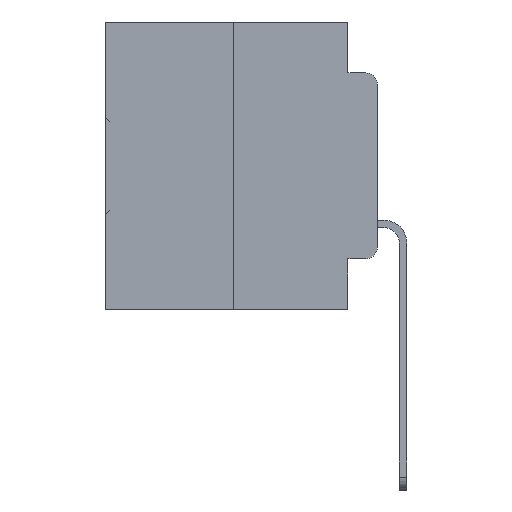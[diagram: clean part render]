
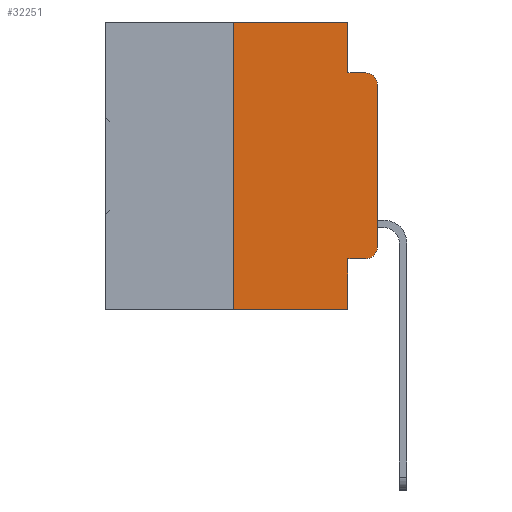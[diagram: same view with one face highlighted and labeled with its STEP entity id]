
A CAD part, left-side view. The second image highlights one B-rep face of the part: STEP entity #32251.
In plain terms, the highlighted planar face has unit normal (-1, 0, 0).
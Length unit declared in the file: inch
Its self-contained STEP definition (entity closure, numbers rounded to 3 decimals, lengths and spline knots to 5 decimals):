
#83 = LINE ( 'NONE', #15399, #19678 ) ;
#830 = ORIENTED_EDGE ( 'NONE', *, *, #25041, .T. ) ;
#836 = CARTESIAN_POINT ( 'NONE',  ( 0., 0.02, -0.3915 ) ) ;
#919 = VERTEX_POINT ( 'NONE', #12145 ) ;
#992 = ORIENTED_EDGE ( 'NONE', *, *, #31967, .T. ) ;
#1198 = VECTOR ( 'NONE', #10958, 39.37008 ) ;
#1769 = EDGE_CURVE ( 'NONE', #11244, #21108, #15442, .T. ) ;
#2056 = DIRECTION ( 'NONE',  ( 0., 0., -1. ) ) ;
#2387 = CARTESIAN_POINT ( 'NONE',  ( 0., 0.051, -0.5 ) ) ;
#3207 = AXIS2_PLACEMENT_3D ( 'NONE', #11219, #29512, #13891 ) ;
#3574 = DIRECTION ( 'NONE',  ( 0., 0., -1. ) ) ;
#4146 = AXIS2_PLACEMENT_3D ( 'NONE', #836, #19469, #3574 ) ;
#4393 = ORIENTED_EDGE ( 'NONE', *, *, #25505, .F. ) ;
#4738 = VECTOR ( 'NONE', #8122, 39.37008 ) ;
#4971 = EDGE_CURVE ( 'NONE', #9365, #25466, #5083, .T. ) ;
#4992 = CARTESIAN_POINT ( 'NONE',  ( 0., 0.051, 0. ) ) ;
#5083 = LINE ( 'NONE', #10403, #18357 ) ;
#5405 = CARTESIAN_POINT ( 'NONE',  ( 0., 0.051, -0.4115 ) ) ;
#8122 = DIRECTION ( 'NONE',  ( 0., -1., 0. ) ) ;
#8273 = CIRCLE ( 'NONE', #4146, 0.02 ) ;
#9365 = VERTEX_POINT ( 'NONE', #17453 ) ;
#10403 = CARTESIAN_POINT ( 'NONE',  ( 0., 0.25, 0. ) ) ;
#10607 = VERTEX_POINT ( 'NONE', #4992 ) ;
#10772 = LINE ( 'NONE', #13073, #17762 ) ;
#10958 = DIRECTION ( 'NONE',  ( 0., 0., 1. ) ) ;
#11066 = EDGE_CURVE ( 'NONE', #9365, #14233, #12855, .T. ) ;
#11219 = CARTESIAN_POINT ( 'NONE',  ( 0., 0.473, 0. ) ) ;
#11244 = VERTEX_POINT ( 'NONE', #16465 ) ;
#11759 = AXIS2_PLACEMENT_3D ( 'NONE', #15131, #33301, #17755 ) ;
#11813 = VECTOR ( 'NONE', #15239, 39.37008 ) ;
#12145 = CARTESIAN_POINT ( 'NONE',  ( 0., 0.02, -0.4115 ) ) ;
#12359 = ORIENTED_EDGE ( 'NONE', *, *, #18378, .F. ) ;
#12530 = CIRCLE ( 'NONE', #11759, 0.02 ) ;
#12855 = LINE ( 'NONE', #20433, #31195 ) ;
#12940 = ORIENTED_EDGE ( 'NONE', *, *, #32003, .F. ) ;
#13073 = CARTESIAN_POINT ( 'NONE',  ( 0., 0.473, 0. ) ) ;
#13258 = EDGE_CURVE ( 'NONE', #10607, #28328, #29925, .T. ) ;
#13891 = DIRECTION ( 'NONE',  ( 0., 0., -1. ) ) ;
#14233 = VERTEX_POINT ( 'NONE', #2387 ) ;
#14582 = ORIENTED_EDGE ( 'NONE', *, *, #1769, .T. ) ;
#15131 = CARTESIAN_POINT ( 'NONE',  ( 0., 0.02, -0.1085 ) ) ;
#15133 = CARTESIAN_POINT ( 'NONE',  ( 0., 0.25, 0. ) ) ;
#15239 = DIRECTION ( 'NONE',  ( 0., -1., 0. ) ) ;
#15251 = VECTOR ( 'NONE', #16353, 39.37008 ) ;
#15399 = CARTESIAN_POINT ( 'NONE',  ( 0., 0.051, 0. ) ) ;
#15442 = LINE ( 'NONE', #21506, #1198 ) ;
#16261 = VERTEX_POINT ( 'NONE', #17396 ) ;
#16353 = DIRECTION ( 'NONE',  ( 0., 0., -1. ) ) ;
#16465 = CARTESIAN_POINT ( 'NONE',  ( 0., 0., -0.3915 ) ) ;
#17396 = CARTESIAN_POINT ( 'NONE',  ( 0., 0.051, -0.4115 ) ) ;
#17453 = CARTESIAN_POINT ( 'NONE',  ( 0., 0.25, -0.5 ) ) ;
#17499 = ORIENTED_EDGE ( 'NONE', *, *, #11066, .T. ) ;
#17755 = DIRECTION ( 'NONE',  ( 0., 0., -1. ) ) ;
#17762 = VECTOR ( 'NONE', #28704, 39.37008 ) ;
#18357 = VECTOR ( 'NONE', #20834, 39.37008 ) ;
#18378 = EDGE_CURVE ( 'NONE', #25466, #10607, #10772, .T. ) ;
#18434 = FACE_OUTER_BOUND ( 'NONE', #30913, .T. ) ;
#19469 = DIRECTION ( 'NONE',  ( -1., 0., 0. ) ) ;
#19678 = VECTOR ( 'NONE', #2056, 39.37008 ) ;
#20121 = ORIENTED_EDGE ( 'NONE', *, *, #4971, .F. ) ;
#20433 = CARTESIAN_POINT ( 'NONE',  ( 0., 0.473, -0.5 ) ) ;
#20779 = ORIENTED_EDGE ( 'NONE', *, *, #23313, .T. ) ;
#20834 = DIRECTION ( 'NONE',  ( 0., 0., 1. ) ) ;
#21108 = VERTEX_POINT ( 'NONE', #25754 ) ;
#21506 = CARTESIAN_POINT ( 'NONE',  ( 0., 0., 0. ) ) ;
#21663 = PLANE ( 'NONE',  #3207 ) ;
#22356 = ORIENTED_EDGE ( 'NONE', *, *, #13258, .F. ) ;
#22930 = DIRECTION ( 'NONE',  ( 0., -1., 0. ) ) ;
#23313 = EDGE_CURVE ( 'NONE', #919, #11244, #8273, .T. ) ;
#24182 = CARTESIAN_POINT ( 'NONE',  ( 0., 0.02, -0.0885 ) ) ;
#25041 = EDGE_CURVE ( 'NONE', #16261, #919, #32653, .T. ) ;
#25466 = VERTEX_POINT ( 'NONE', #15133 ) ;
#25505 = EDGE_CURVE ( 'NONE', #28328, #30477, #31829, .T. ) ;
#25754 = CARTESIAN_POINT ( 'NONE',  ( 0., 0., -0.1085 ) ) ;
#28328 = VERTEX_POINT ( 'NONE', #32844 ) ;
#28704 = DIRECTION ( 'NONE',  ( 0., -1., 0. ) ) ;
#29337 = CARTESIAN_POINT ( 'NONE',  ( 0., 0.051, 0. ) ) ;
#29512 = DIRECTION ( 'NONE',  ( 1., 0., 0. ) ) ;
#29925 = LINE ( 'NONE', #29337, #15251 ) ;
#30477 = VERTEX_POINT ( 'NONE', #24182 ) ;
#30913 = EDGE_LOOP ( 'NONE', ( #14582, #992, #4393, #22356, #12359, #20121, #17499, #12940, #830, #20779 ) ) ;
#31195 = VECTOR ( 'NONE', #22930, 39.37008 ) ;
#31829 = LINE ( 'NONE', #33406, #11813 ) ;
#31967 = EDGE_CURVE ( 'NONE', #21108, #30477, #12530, .T. ) ;
#32003 = EDGE_CURVE ( 'NONE', #16261, #14233, #83, .T. ) ;
#32251 = ADVANCED_FACE ( 'NONE', ( #18434 ), #21663, .F. ) ;
#32653 = LINE ( 'NONE', #5405, #4738 ) ;
#32844 = CARTESIAN_POINT ( 'NONE',  ( 0., 0.051, -0.0885 ) ) ;
#33301 = DIRECTION ( 'NONE',  ( -1., 0., 0. ) ) ;
#33406 = CARTESIAN_POINT ( 'NONE',  ( 0., 0.051, -0.0885 ) ) ;
